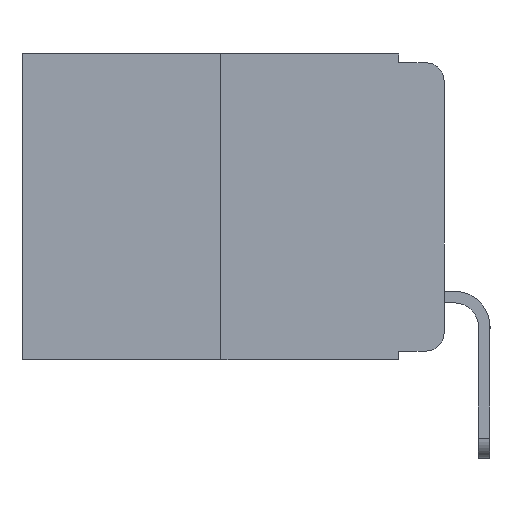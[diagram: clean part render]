
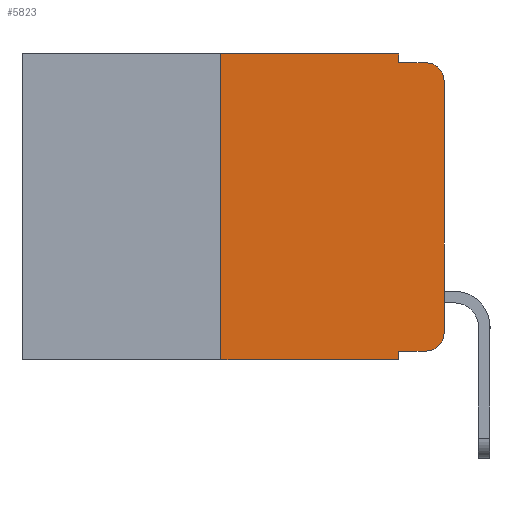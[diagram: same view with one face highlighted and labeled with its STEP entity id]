
A CAD part, left-side view. The second image highlights one B-rep face of the part: STEP entity #5823.
In plain terms, the highlighted planar face has unit normal (-1, 0, 0).
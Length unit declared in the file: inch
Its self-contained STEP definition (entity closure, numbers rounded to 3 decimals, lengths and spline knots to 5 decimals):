
#267 = ORIENTED_EDGE ( 'NONE', *, *, #1207, .F. ) ;
#431 = ORIENTED_EDGE ( 'NONE', *, *, #1553, .T. ) ;
#546 = DIRECTION ( 'NONE',  ( 0., 0., 1. ) ) ;
#705 = ORIENTED_EDGE ( 'NONE', *, *, #1139, .T. ) ;
#839 = VERTEX_POINT ( 'NONE', #7415 ) ;
#1093 = EDGE_CURVE ( 'NONE', #3534, #4471, #10159, .T. ) ;
#1095 = CIRCLE ( 'NONE', #7885, 0.02 ) ;
#1139 = EDGE_CURVE ( 'NONE', #4471, #1381, #5155, .T. ) ;
#1207 = EDGE_CURVE ( 'NONE', #2592, #1381, #9040, .T. ) ;
#1270 = EDGE_CURVE ( 'NONE', #839, #2592, #8789, .T. ) ;
#1381 = VERTEX_POINT ( 'NONE', #12164 ) ;
#1407 = EDGE_CURVE ( 'NONE', #8210, #3206, #9748, .T. ) ;
#1521 = CARTESIAN_POINT ( 'NONE',  ( 0., 0., 0. ) ) ;
#1532 = EDGE_CURVE ( 'NONE', #5328, #7078, #9179, .T. ) ;
#1553 = EDGE_CURVE ( 'NONE', #5328, #2890, #3378, .T. ) ;
#1682 = EDGE_CURVE ( 'NONE', #2890, #3534, #1095, .T. ) ;
#2415 = ORIENTED_EDGE ( 'NONE', *, *, #1407, .F. ) ;
#2532 = ORIENTED_EDGE ( 'NONE', *, *, #1532, .F. ) ;
#2592 = VERTEX_POINT ( 'NONE', #12615 ) ;
#2890 = VERTEX_POINT ( 'NONE', #11951 ) ;
#3132 = EDGE_LOOP ( 'NONE', ( #4989, #705, #267, #4821, #4353, #2415, #4219, #2532, #431, #9711 ) ) ;
#3206 = VERTEX_POINT ( 'NONE', #11389 ) ;
#3378 = LINE ( 'NONE', #12268, #10687 ) ;
#3534 = VERTEX_POINT ( 'NONE', #12343 ) ;
#3745 = CARTESIAN_POINT ( 'NONE',  ( 0., 0.473, 0. ) ) ;
#3807 = VECTOR ( 'NONE', #12069, 39.37008 ) ;
#4219 = ORIENTED_EDGE ( 'NONE', *, *, #8804, .T. ) ;
#4251 = DIRECTION ( 'NONE',  ( 0., 0., -1. ) ) ;
#4337 = DIRECTION ( 'NONE',  ( 0., -1., 0. ) ) ;
#4353 = ORIENTED_EDGE ( 'NONE', *, *, #10554, .F. ) ;
#4471 = VERTEX_POINT ( 'NONE', #8699 ) ;
#4591 = VECTOR ( 'NONE', #4337, 39.37008 ) ;
#4619 = VECTOR ( 'NONE', #546, 39.37008 ) ;
#4751 = CARTESIAN_POINT ( 'NONE',  ( 0., 0.25, 0. ) ) ;
#4821 = ORIENTED_EDGE ( 'NONE', *, *, #1270, .F. ) ;
#4989 = ORIENTED_EDGE ( 'NONE', *, *, #1093, .T. ) ;
#5155 = CIRCLE ( 'NONE', #12184, 0.02 ) ;
#5215 = DIRECTION ( 'NONE',  ( -1., 0., 0. ) ) ;
#5328 = VERTEX_POINT ( 'NONE', #11365 ) ;
#5751 = LINE ( 'NONE', #3745, #10094 ) ;
#5823 = ADVANCED_FACE ( 'NONE', ( #8831 ), #9857, .F. ) ;
#5888 = DIRECTION ( 'NONE',  ( 0., 0., -1. ) ) ;
#6799 = CARTESIAN_POINT ( 'NONE',  ( 0., 0.02, -0.313 ) ) ;
#6957 = CARTESIAN_POINT ( 'NONE',  ( 0., 0.051, 0. ) ) ;
#7078 = VERTEX_POINT ( 'NONE', #12396 ) ;
#7211 = DIRECTION ( 'NONE',  ( 0., 0., 1. ) ) ;
#7415 = CARTESIAN_POINT ( 'NONE',  ( 0., 0.051, 0. ) ) ;
#7850 = VECTOR ( 'NONE', #7211, 39.37008 ) ;
#7885 = AXIS2_PLACEMENT_3D ( 'NONE', #6799, #5215, #4251 ) ;
#7893 = DIRECTION ( 'NONE',  ( 0., -1., 0. ) ) ;
#7966 = CARTESIAN_POINT ( 'NONE',  ( 0., 0.02, -0.03 ) ) ;
#8210 = VERTEX_POINT ( 'NONE', #10020 ) ;
#8252 = VECTOR ( 'NONE', #9219, 39.37008 ) ;
#8653 = VECTOR ( 'NONE', #5888, 39.37008 ) ;
#8699 = CARTESIAN_POINT ( 'NONE',  ( 0., 0., -0.03 ) ) ;
#8789 = LINE ( 'NONE', #9004, #8252 ) ;
#8804 = EDGE_CURVE ( 'NONE', #8210, #7078, #12324, .T. ) ;
#8831 = FACE_OUTER_BOUND ( 'NONE', #3132, .T. ) ;
#9004 = CARTESIAN_POINT ( 'NONE',  ( 0., 0.051, 0. ) ) ;
#9040 = LINE ( 'NONE', #10343, #3807 ) ;
#9133 = AXIS2_PLACEMENT_3D ( 'NONE', #9697, #9824, #9918 ) ;
#9179 = LINE ( 'NONE', #6957, #8653 ) ;
#9219 = DIRECTION ( 'NONE',  ( 0., 0., -1. ) ) ;
#9697 = CARTESIAN_POINT ( 'NONE',  ( 0., 0.473, 0. ) ) ;
#9711 = ORIENTED_EDGE ( 'NONE', *, *, #1682, .T. ) ;
#9748 = LINE ( 'NONE', #4751, #4619 ) ;
#9824 = DIRECTION ( 'NONE',  ( 1., 0., 0. ) ) ;
#9857 = PLANE ( 'NONE',  #9133 ) ;
#9918 = DIRECTION ( 'NONE',  ( 0., 0., -1. ) ) ;
#10020 = CARTESIAN_POINT ( 'NONE',  ( 0., 0.25, -0.343 ) ) ;
#10094 = VECTOR ( 'NONE', #7893, 39.37008 ) ;
#10159 = LINE ( 'NONE', #1521, #7850 ) ;
#10343 = CARTESIAN_POINT ( 'NONE',  ( 0., 0.051, -0.01 ) ) ;
#10464 = DIRECTION ( 'NONE',  ( 0., -1., 0. ) ) ;
#10554 = EDGE_CURVE ( 'NONE', #3206, #839, #5751, .T. ) ;
#10687 = VECTOR ( 'NONE', #10464, 39.37008 ) ;
#11209 = DIRECTION ( 'NONE',  ( 0., 0., -1. ) ) ;
#11365 = CARTESIAN_POINT ( 'NONE',  ( 0., 0.051, -0.333 ) ) ;
#11389 = CARTESIAN_POINT ( 'NONE',  ( 0., 0.25, 0. ) ) ;
#11951 = CARTESIAN_POINT ( 'NONE',  ( 0., 0.02, -0.333 ) ) ;
#12069 = DIRECTION ( 'NONE',  ( 0., -1., 0. ) ) ;
#12164 = CARTESIAN_POINT ( 'NONE',  ( 0., 0.02, -0.01 ) ) ;
#12184 = AXIS2_PLACEMENT_3D ( 'NONE', #7966, #12591, #11209 ) ;
#12268 = CARTESIAN_POINT ( 'NONE',  ( 0., 0.051, -0.333 ) ) ;
#12324 = LINE ( 'NONE', #12566, #4591 ) ;
#12343 = CARTESIAN_POINT ( 'NONE',  ( 0., 0., -0.313 ) ) ;
#12396 = CARTESIAN_POINT ( 'NONE',  ( 0., 0.051, -0.343 ) ) ;
#12566 = CARTESIAN_POINT ( 'NONE',  ( 0., 0.473, -0.343 ) ) ;
#12591 = DIRECTION ( 'NONE',  ( -1., 0., 0. ) ) ;
#12615 = CARTESIAN_POINT ( 'NONE',  ( 0., 0.051, -0.01 ) ) ;
